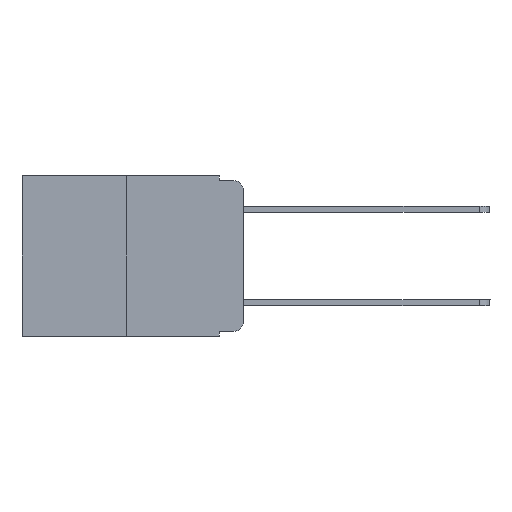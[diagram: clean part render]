
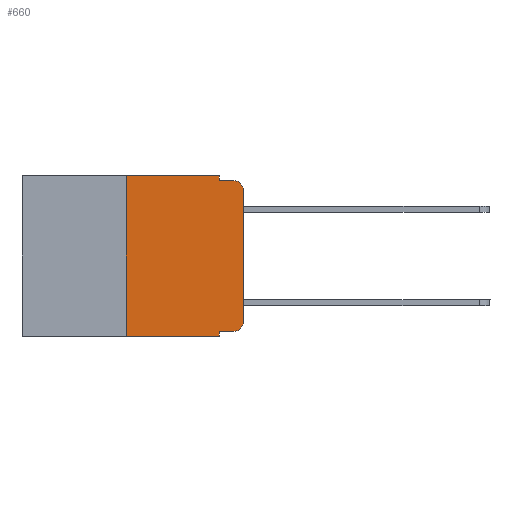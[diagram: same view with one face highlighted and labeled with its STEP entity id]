
A CAD part, left-side view. The second image highlights one B-rep face of the part: STEP entity #660.
In plain terms, the highlighted planar face has unit normal (-1, 0, 0).
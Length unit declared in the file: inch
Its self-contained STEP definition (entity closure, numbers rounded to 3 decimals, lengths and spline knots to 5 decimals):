
#129 = CIRCLE ( 'NONE', #767, 0.02 ) ;
#390 = EDGE_CURVE ( 'NONE', #4237, #2374, #129, .T. ) ;
#453 = EDGE_CURVE ( 'NONE', #1510, #3737, #5525, .T. ) ;
#592 = DIRECTION ( 'NONE',  ( 0., -1., 0. ) ) ;
#660 = ADVANCED_FACE ( 'NONE', ( #1409 ), #8294, .F. ) ;
#672 = LINE ( 'NONE', #4404, #3062 ) ;
#726 = ORIENTED_EDGE ( 'NONE', *, *, #3498, .F. ) ;
#736 = ORIENTED_EDGE ( 'NONE', *, *, #8749, .T. ) ;
#767 = AXIS2_PLACEMENT_3D ( 'NONE', #8367, #1573, #850 ) ;
#792 = CARTESIAN_POINT ( 'NONE',  ( 0., 0.473, 0. ) ) ;
#838 = VECTOR ( 'NONE', #8288, 39.37008 ) ;
#850 = DIRECTION ( 'NONE',  ( 0., 0., -1. ) ) ;
#982 = VECTOR ( 'NONE', #5993, 39.37008 ) ;
#1162 = VECTOR ( 'NONE', #8535, 39.37008 ) ;
#1401 = CARTESIAN_POINT ( 'NONE',  ( 0., 0.02, -0.03 ) ) ;
#1409 = FACE_OUTER_BOUND ( 'NONE', #9310, .T. ) ;
#1466 = LINE ( 'NONE', #3027, #4084 ) ;
#1510 = VERTEX_POINT ( 'NONE', #7215 ) ;
#1573 = DIRECTION ( 'NONE',  ( -1., 0., 0. ) ) ;
#1932 = EDGE_CURVE ( 'NONE', #2374, #2886, #5518, .T. ) ;
#2203 = VECTOR ( 'NONE', #5111, 39.37008 ) ;
#2252 = CARTESIAN_POINT ( 'NONE',  ( 0., 0.051, 0. ) ) ;
#2257 = ORIENTED_EDGE ( 'NONE', *, *, #1932, .T. ) ;
#2374 = VERTEX_POINT ( 'NONE', #4027 ) ;
#2581 = VECTOR ( 'NONE', #7809, 39.37008 ) ;
#2794 = DIRECTION ( 'NONE',  ( -1., 0., 0. ) ) ;
#2886 = VERTEX_POINT ( 'NONE', #8426 ) ;
#3018 = EDGE_CURVE ( 'NONE', #3457, #3113, #7759, .T. ) ;
#3027 = CARTESIAN_POINT ( 'NONE',  ( 0., 0.051, -0.333 ) ) ;
#3062 = VECTOR ( 'NONE', #3679, 39.37008 ) ;
#3113 = VERTEX_POINT ( 'NONE', #3628 ) ;
#3210 = CARTESIAN_POINT ( 'NONE',  ( 0., 0., 0. ) ) ;
#3304 = VERTEX_POINT ( 'NONE', #4498 ) ;
#3457 = VERTEX_POINT ( 'NONE', #3604 ) ;
#3498 = EDGE_CURVE ( 'NONE', #3304, #9449, #7452, .T. ) ;
#3604 = CARTESIAN_POINT ( 'NONE',  ( 0., 0.25, -0.343 ) ) ;
#3628 = CARTESIAN_POINT ( 'NONE',  ( 0., 0.051, -0.343 ) ) ;
#3679 = DIRECTION ( 'NONE',  ( 0., 0., -1. ) ) ;
#3682 = AXIS2_PLACEMENT_3D ( 'NONE', #1401, #2794, #8036 ) ;
#3737 = VERTEX_POINT ( 'NONE', #7975 ) ;
#4027 = CARTESIAN_POINT ( 'NONE',  ( 0., 0., -0.313 ) ) ;
#4084 = VECTOR ( 'NONE', #5270, 39.37008 ) ;
#4237 = VERTEX_POINT ( 'NONE', #4990 ) ;
#4404 = CARTESIAN_POINT ( 'NONE',  ( 0., 0.051, 0. ) ) ;
#4422 = DIRECTION ( 'NONE',  ( 0., 0., -1. ) ) ;
#4483 = VERTEX_POINT ( 'NONE', #7426 ) ;
#4498 = CARTESIAN_POINT ( 'NONE',  ( 0., 0.25, 0. ) ) ;
#4792 = CARTESIAN_POINT ( 'NONE',  ( 0., 0.473, -0.343 ) ) ;
#4990 = CARTESIAN_POINT ( 'NONE',  ( 0., 0.02, -0.333 ) ) ;
#5111 = DIRECTION ( 'NONE',  ( 0., 0., 1. ) ) ;
#5270 = DIRECTION ( 'NONE',  ( 0., -1., 0. ) ) ;
#5392 = LINE ( 'NONE', #6645, #2203 ) ;
#5518 = LINE ( 'NONE', #3210, #1162 ) ;
#5525 = LINE ( 'NONE', #6260, #9415 ) ;
#5531 = ORIENTED_EDGE ( 'NONE', *, *, #6268, .F. ) ;
#5745 = ORIENTED_EDGE ( 'NONE', *, *, #9149, .F. ) ;
#5750 = ORIENTED_EDGE ( 'NONE', *, *, #453, .F. ) ;
#5789 = EDGE_CURVE ( 'NONE', #9449, #1510, #672, .T. ) ;
#5894 = DIRECTION ( 'NONE',  ( 1., 0., 0. ) ) ;
#5993 = DIRECTION ( 'NONE',  ( 0., -1., 0. ) ) ;
#6130 = EDGE_CURVE ( 'NONE', #2886, #3737, #7126, .T. ) ;
#6260 = CARTESIAN_POINT ( 'NONE',  ( 0., 0.051, -0.01 ) ) ;
#6268 = EDGE_CURVE ( 'NONE', #4483, #3113, #9112, .T. ) ;
#6645 = CARTESIAN_POINT ( 'NONE',  ( 0., 0.25, 0. ) ) ;
#7126 = CIRCLE ( 'NONE', #3682, 0.02 ) ;
#7215 = CARTESIAN_POINT ( 'NONE',  ( 0., 0.051, -0.01 ) ) ;
#7426 = CARTESIAN_POINT ( 'NONE',  ( 0., 0.051, -0.333 ) ) ;
#7443 = ORIENTED_EDGE ( 'NONE', *, *, #6130, .T. ) ;
#7452 = LINE ( 'NONE', #792, #982 ) ;
#7759 = LINE ( 'NONE', #4792, #2581 ) ;
#7809 = DIRECTION ( 'NONE',  ( 0., -1., 0. ) ) ;
#7975 = CARTESIAN_POINT ( 'NONE',  ( 0., 0.02, -0.01 ) ) ;
#8036 = DIRECTION ( 'NONE',  ( 0., 0., -1. ) ) ;
#8147 = ORIENTED_EDGE ( 'NONE', *, *, #5789, .F. ) ;
#8178 = ORIENTED_EDGE ( 'NONE', *, *, #3018, .T. ) ;
#8288 = DIRECTION ( 'NONE',  ( 0., 0., -1. ) ) ;
#8294 = PLANE ( 'NONE',  #9228 ) ;
#8367 = CARTESIAN_POINT ( 'NONE',  ( 0., 0.02, -0.313 ) ) ;
#8426 = CARTESIAN_POINT ( 'NONE',  ( 0., 0., -0.03 ) ) ;
#8535 = DIRECTION ( 'NONE',  ( 0., 0., 1. ) ) ;
#8749 = EDGE_CURVE ( 'NONE', #4483, #4237, #1466, .T. ) ;
#8802 = CARTESIAN_POINT ( 'NONE',  ( 0., 0.051, 0. ) ) ;
#8925 = CARTESIAN_POINT ( 'NONE',  ( 0., 0.473, 0. ) ) ;
#9112 = LINE ( 'NONE', #2252, #838 ) ;
#9149 = EDGE_CURVE ( 'NONE', #3457, #3304, #5392, .T. ) ;
#9228 = AXIS2_PLACEMENT_3D ( 'NONE', #8925, #5894, #4422 ) ;
#9310 = EDGE_LOOP ( 'NONE', ( #2257, #7443, #5750, #8147, #726, #5745, #8178, #5531, #736, #9749 ) ) ;
#9415 = VECTOR ( 'NONE', #592, 39.37008 ) ;
#9449 = VERTEX_POINT ( 'NONE', #8802 ) ;
#9749 = ORIENTED_EDGE ( 'NONE', *, *, #390, .T. ) ;
